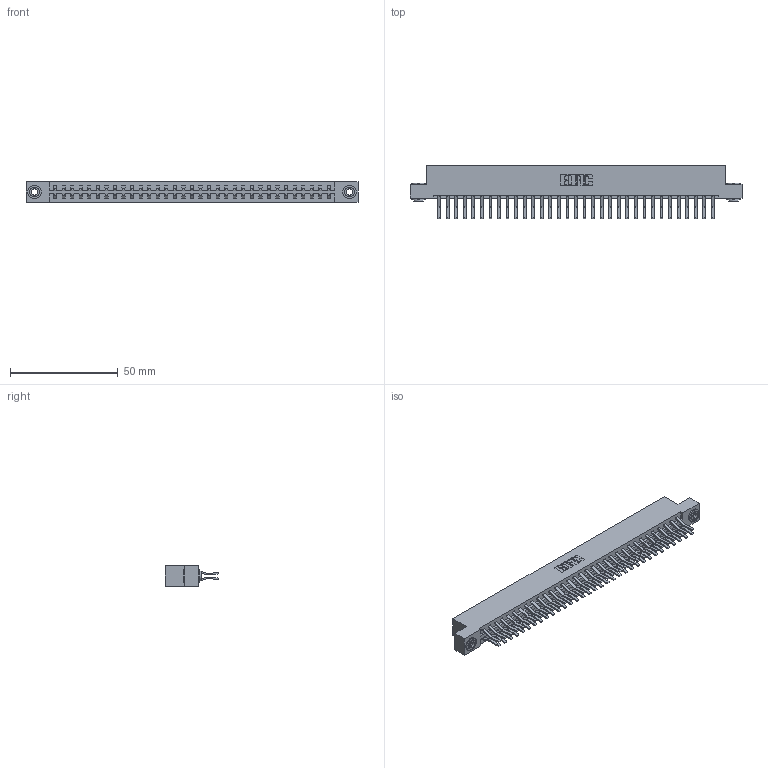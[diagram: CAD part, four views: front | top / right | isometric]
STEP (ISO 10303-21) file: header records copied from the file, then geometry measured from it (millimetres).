
FILE_DESCRIPTION (( 'STEP AP203' ), '1' );
FILE_NAME ('337-066-560-203.STEP', '2018-08-11T08:57:15', ( '' ), ( '' ), 'SwSTEP 2.0', 'SolidWorks 2016', '' );
FILE_SCHEMA (( 'CONFIG_CONTROL_DESIGN' ));
Length unit declared in the file: inch
Products named in the file (4): 337 Part_Flush Mounting Lugs - 0.156 Dia-TH; 345-292-001_560 Tail; 345-250-002_345-250-002-102; 337-066-560-203
Assembly tree (69 placements, depth 2):
  337-066-560-203
    337 Part_Flush Mounting Lugs - 0.156 Dia-TH
    345-292-001_560 Tail  x66
    345-250-002_345-250-002-102  x2
Bounding box: 153.77 x 24.78 x 9.4 mm (x, y, z)
Volume: 16537.9 mm3; surface area: 20085.1 mm2
Topology: 69 solids, 69 shells, 3848 faces, 11409 edges, 7514 vertices
Faces by surface type: plane 2588, cylinder 1252, cone 8
Entity records: 27488 total; most frequent: CARTESIAN_POINT 4613, ORIENTED_EDGE 4542, DIRECTION 3977, EDGE_CURVE 2271, VECTOR 2115, LINE 2115, VERTEX_POINT 1510, AXIS2_PLACEMENT_3D 931
